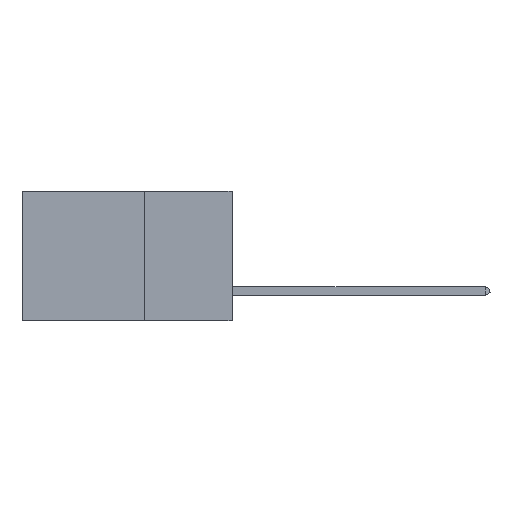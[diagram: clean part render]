
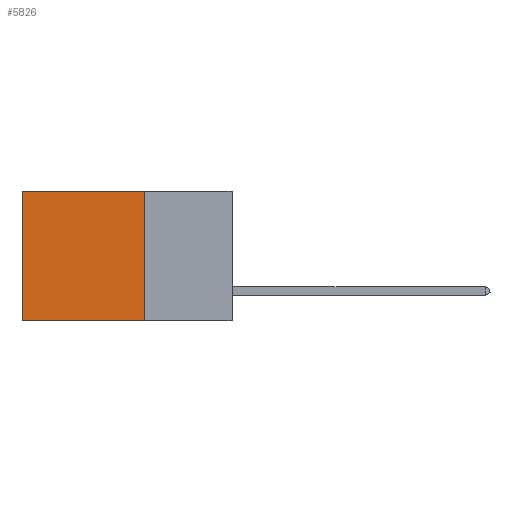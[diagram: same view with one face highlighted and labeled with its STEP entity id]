
A CAD part, left-side view. The second image highlights one B-rep face of the part: STEP entity #5826.
In plain terms, the highlighted planar face has unit normal (-1, 0, 0).
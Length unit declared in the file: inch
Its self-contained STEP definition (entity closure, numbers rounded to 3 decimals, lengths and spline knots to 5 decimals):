
#423 = EDGE_CURVE ( 'NONE', #1479, #14495, #7198, .T. ) ;
#1479 = VERTEX_POINT ( 'NONE', #1526 ) ;
#1501 = CARTESIAN_POINT ( 'NONE',  ( 0.2875, 0.6, 0. ) ) ;
#1526 = CARTESIAN_POINT ( 'NONE',  ( 0.2875, 0.25, 0. ) ) ;
#1791 = CARTESIAN_POINT ( 'NONE',  ( 0.2875, 0.25, -0.37 ) ) ;
#1893 = DIRECTION ( 'NONE',  ( 0., 1., 0. ) ) ;
#1962 = DIRECTION ( 'NONE',  ( 0., 0., -1. ) ) ;
#2795 = VERTEX_POINT ( 'NONE', #6809 ) ;
#2833 = EDGE_CURVE ( 'NONE', #15723, #2795, #3162, .T. ) ;
#3162 = LINE ( 'NONE', #12413, #13497 ) ;
#3932 = VECTOR ( 'NONE', #1962, 39.37008 ) ;
#4013 = ORIENTED_EDGE ( 'NONE', *, *, #7675, .T. ) ;
#4877 = EDGE_CURVE ( 'NONE', #1479, #15723, #7870, .T. ) ;
#5826 = ADVANCED_FACE ( 'NONE', ( #7836 ), #10698, .F. ) ;
#6299 = AXIS2_PLACEMENT_3D ( 'NONE', #7001, #10934, #12207 ) ;
#6355 = EDGE_LOOP ( 'NONE', ( #4013, #11539, #15063, #7236 ) ) ;
#6479 = CARTESIAN_POINT ( 'NONE',  ( 0.2875, 0.25, 0. ) ) ;
#6602 = DIRECTION ( 'NONE',  ( 0., 1., 0. ) ) ;
#6809 = CARTESIAN_POINT ( 'NONE',  ( 0.2875, 0.6, -0.37 ) ) ;
#7001 = CARTESIAN_POINT ( 'NONE',  ( 0.2875, 0.25, 0. ) ) ;
#7198 = LINE ( 'NONE', #14419, #11493 ) ;
#7236 = ORIENTED_EDGE ( 'NONE', *, *, #423, .T. ) ;
#7455 = LINE ( 'NONE', #13935, #3932 ) ;
#7675 = EDGE_CURVE ( 'NONE', #14495, #2795, #7455, .T. ) ;
#7836 = FACE_OUTER_BOUND ( 'NONE', #6355, .T. ) ;
#7870 = LINE ( 'NONE', #6479, #9322 ) ;
#9322 = VECTOR ( 'NONE', #14413, 39.37008 ) ;
#10698 = PLANE ( 'NONE',  #6299 ) ;
#10934 = DIRECTION ( 'NONE',  ( 1., 0., 0. ) ) ;
#11493 = VECTOR ( 'NONE', #6602, 39.37008 ) ;
#11539 = ORIENTED_EDGE ( 'NONE', *, *, #2833, .F. ) ;
#12207 = DIRECTION ( 'NONE',  ( 0., 0., -1. ) ) ;
#12413 = CARTESIAN_POINT ( 'NONE',  ( 0.2875, 0.25, -0.37 ) ) ;
#13497 = VECTOR ( 'NONE', #1893, 39.37008 ) ;
#13935 = CARTESIAN_POINT ( 'NONE',  ( 0.2875, 0.6, 0. ) ) ;
#14413 = DIRECTION ( 'NONE',  ( 0., 0., -1. ) ) ;
#14419 = CARTESIAN_POINT ( 'NONE',  ( 0.2875, 0.25, 0. ) ) ;
#14495 = VERTEX_POINT ( 'NONE', #1501 ) ;
#15063 = ORIENTED_EDGE ( 'NONE', *, *, #4877, .F. ) ;
#15723 = VERTEX_POINT ( 'NONE', #1791 ) ;
